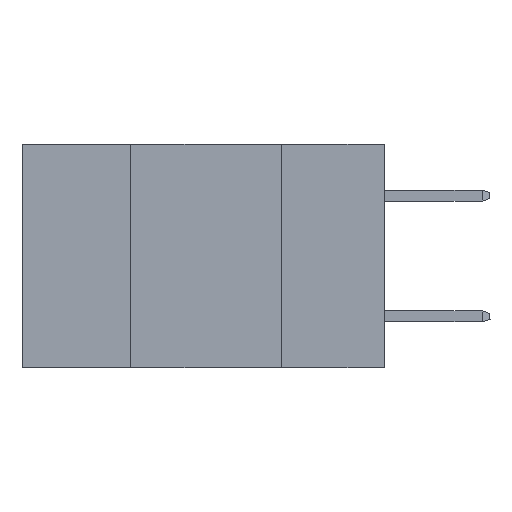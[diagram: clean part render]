
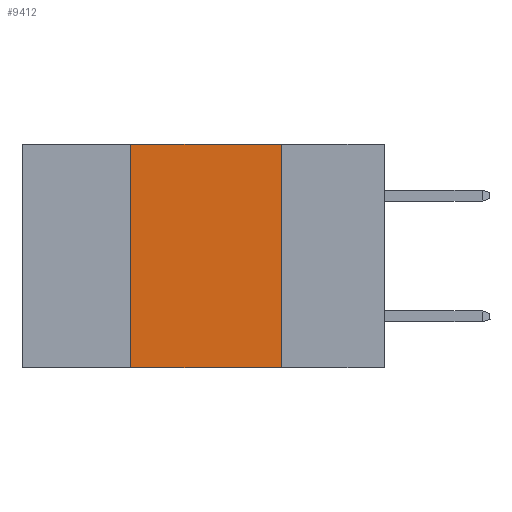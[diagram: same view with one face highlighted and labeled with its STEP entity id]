
A CAD part, left-side view. The second image highlights one B-rep face of the part: STEP entity #9412.
In plain terms, the highlighted planar face has unit normal (-1, 0, 0).
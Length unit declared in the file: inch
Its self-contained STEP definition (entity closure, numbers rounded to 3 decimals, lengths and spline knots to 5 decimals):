
#594 = DIRECTION ( 'NONE',  ( 0., 0., -1. ) ) ;
#711 = CARTESIAN_POINT ( 'NONE',  ( 0., 0.17, -0.37 ) ) ;
#1636 = CARTESIAN_POINT ( 'NONE',  ( 0., 0.17, 0. ) ) ;
#1814 = EDGE_CURVE ( 'NONE', #13118, #7636, #3648, .T. ) ;
#1846 = CARTESIAN_POINT ( 'NONE',  ( 0., 0.42, -0.37 ) ) ;
#2026 = ORIENTED_EDGE ( 'NONE', *, *, #1814, .F. ) ;
#2353 = CARTESIAN_POINT ( 'NONE',  ( 0., 0.6, 0. ) ) ;
#2753 = FACE_OUTER_BOUND ( 'NONE', #13272, .T. ) ;
#3648 = LINE ( 'NONE', #8009, #13983 ) ;
#4298 = ORIENTED_EDGE ( 'NONE', *, *, #4576, .F. ) ;
#4450 = VECTOR ( 'NONE', #15399, 39.37008 ) ;
#4534 = ORIENTED_EDGE ( 'NONE', *, *, #5466, .F. ) ;
#4576 = EDGE_CURVE ( 'NONE', #7636, #15540, #8448, .T. ) ;
#5466 = EDGE_CURVE ( 'NONE', #15540, #12725, #8415, .T. ) ;
#6453 = PLANE ( 'NONE',  #14116 ) ;
#7511 = LINE ( 'NONE', #8582, #11105 ) ;
#7636 = VERTEX_POINT ( 'NONE', #15094 ) ;
#7812 = DIRECTION ( 'NONE',  ( 0., 0., -1. ) ) ;
#7986 = VECTOR ( 'NONE', #594, 39.37008 ) ;
#8009 = CARTESIAN_POINT ( 'NONE',  ( 0., 0.42, -0.37 ) ) ;
#8415 = LINE ( 'NONE', #711, #7986 ) ;
#8448 = LINE ( 'NONE', #13733, #4450 ) ;
#8582 = CARTESIAN_POINT ( 'NONE',  ( 0., 0.6, -0.37 ) ) ;
#9412 = ADVANCED_FACE ( 'NONE', ( #2753 ), #6453, .F. ) ;
#11105 = VECTOR ( 'NONE', #16566, 39.37008 ) ;
#11923 = CARTESIAN_POINT ( 'NONE',  ( 0., 0.17, -0.37 ) ) ;
#12652 = ORIENTED_EDGE ( 'NONE', *, *, #17423, .T. ) ;
#12725 = VERTEX_POINT ( 'NONE', #11923 ) ;
#13118 = VERTEX_POINT ( 'NONE', #1846 ) ;
#13272 = EDGE_LOOP ( 'NONE', ( #4534, #4298, #2026, #12652 ) ) ;
#13733 = CARTESIAN_POINT ( 'NONE',  ( 0., 0.6, 0. ) ) ;
#13983 = VECTOR ( 'NONE', #16069, 39.37008 ) ;
#14116 = AXIS2_PLACEMENT_3D ( 'NONE', #2353, #15829, #7812 ) ;
#15094 = CARTESIAN_POINT ( 'NONE',  ( 0., 0.42, 0. ) ) ;
#15399 = DIRECTION ( 'NONE',  ( 0., -1., 0. ) ) ;
#15540 = VERTEX_POINT ( 'NONE', #1636 ) ;
#15829 = DIRECTION ( 'NONE',  ( 1., 0., 0. ) ) ;
#16069 = DIRECTION ( 'NONE',  ( 0., 0., 1. ) ) ;
#16566 = DIRECTION ( 'NONE',  ( 0., -1., 0. ) ) ;
#17423 = EDGE_CURVE ( 'NONE', #13118, #12725, #7511, .T. ) ;
